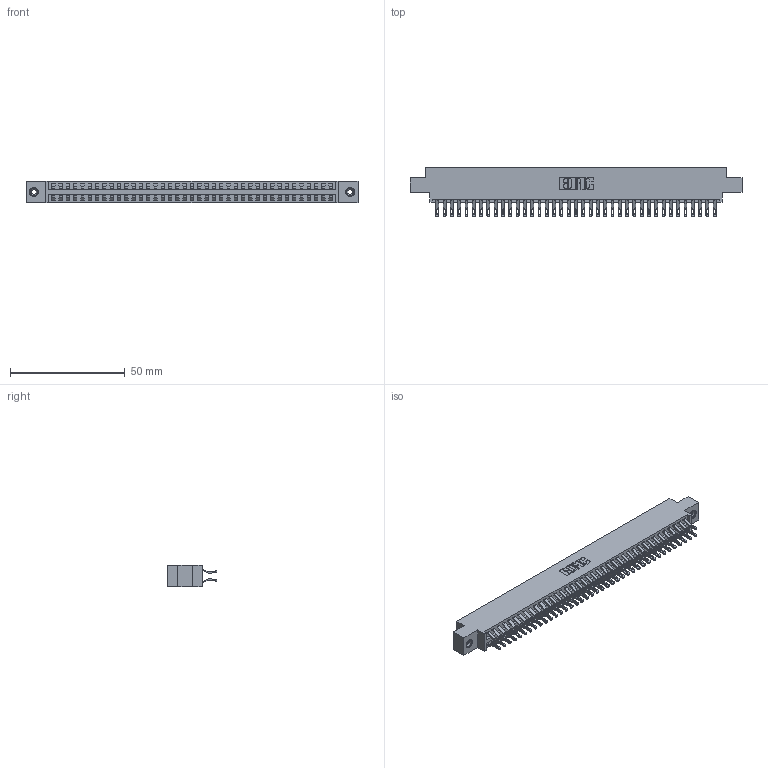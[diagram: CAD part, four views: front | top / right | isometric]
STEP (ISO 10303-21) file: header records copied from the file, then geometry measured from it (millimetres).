
FILE_DESCRIPTION (( 'STEP AP203' ), '1' );
FILE_NAME ('396-078-555-808.STEP', '2019-11-02T13:25:35', ( '' ), ( '' ), 'SwSTEP 2.0', 'SolidWorks 2016', '' );
FILE_SCHEMA (( 'CONFIG_CONTROL_DESIGN' ));
Length unit declared in the file: inch
Products named in the file (4): 346 Part_0.170 Offset - 0.156 Dia-TI; 345-292-001_555 Tail; 345-250-001_345-250-003-102; 396-078-555-808
Assembly tree (81 placements, depth 2):
  396-078-555-808
    346 Part_0.170 Offset - 0.156 Dia-TI
    345-292-001_555 Tail  x78
    345-250-001_345-250-003-102  x2
Bounding box: 144.4 x 21.46 x 9.4 mm (x, y, z)
Volume: 14122.5 mm3; surface area: 20371.3 mm2
Topology: 81 solids, 81 shells, 4710 faces, 14751 edges, 9826 vertices
Faces by surface type: plane 2686, cylinder 2008, cone 12, torus 4
Entity records: 27500 total; most frequent: CARTESIAN_POINT 4557, ORIENTED_EDGE 4454, DIRECTION 4061, EDGE_CURVE 2227, LINE 1899, VECTOR 1899, VERTEX_POINT 1480, AXIS2_PLACEMENT_3D 1081
